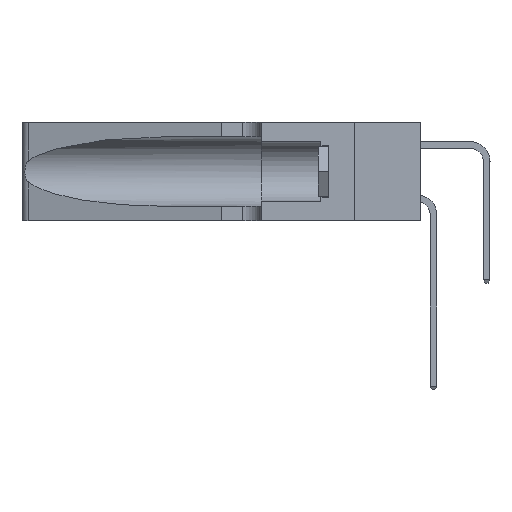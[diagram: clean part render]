
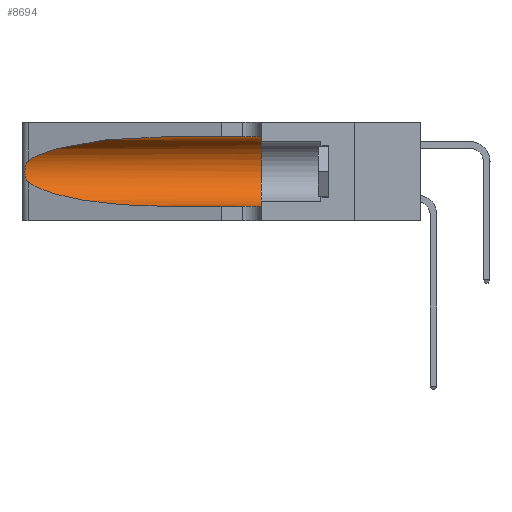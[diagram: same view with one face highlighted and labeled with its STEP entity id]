
A CAD part, left-side view. The second image highlights one B-rep face of the part: STEP entity #8694.
In plain terms, the highlighted cylindrical face has radius 3.308 mm (diameter 6.617 mm), a partial arc.
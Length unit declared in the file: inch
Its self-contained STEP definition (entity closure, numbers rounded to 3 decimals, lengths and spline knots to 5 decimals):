
#302 = EDGE_CURVE ( 'NONE', #23426, #15752, #14535, .T. ) ;
#501 = CARTESIAN_POINT ( 'NONE',  ( 0.18966, 0.96281, 0.31525 ) ) ;
#1126 = CARTESIAN_POINT ( 'NONE',  ( 0.25555, 1.22994, 0.2215 ) ) ;
#1220 = CARTESIAN_POINT ( 'NONE',  ( 0.25854, 1.2359, 0.20912 ) ) ;
#1507 = VECTOR ( 'NONE', #12776, 39.37008 ) ;
#2389 =( BOUNDED_CURVE ( )  B_SPLINE_CURVE ( 3, ( #27854, #23503, #28243, #2604 ),
 .UNSPECIFIED., .F., .T. ) 
 B_SPLINE_CURVE_WITH_KNOTS ( ( 4, 4 ),
 ( 3.44316, 4.71239 ),
 .UNSPECIFIED. ) 
 CURVE ( )  GEOMETRIC_REPRESENTATION_ITEM ( )  RATIONAL_B_SPLINE_CURVE ( ( 1., 0.87, 0.87, 1. ) ) 
 REPRESENTATION_ITEM ( '' )  );
#2604 = CARTESIAN_POINT ( 'NONE',  ( 0.1305, 0.72297, 0.05475 ) ) ;
#2962 = CARTESIAN_POINT ( 'NONE',  ( 0.1305, 0.72297, 0.31525 ) ) ;
#2973 = CYLINDRICAL_SURFACE ( 'NONE', #15668, 0.13025 ) ;
#3079 = CARTESIAN_POINT ( 'NONE',  ( 0.1305, 1.61858, 0.05475 ) ) ;
#3921 = EDGE_LOOP ( 'NONE', ( #8432, #19907, #19055, #15913, #11476, #18027 ) ) ;
#5424 = CARTESIAN_POINT ( 'NONE',  ( 0.25487, 1.22718, 0.22369 ) ) ;
#6348 = EDGE_CURVE ( 'NONE', #6691, #15752, #23844, .T. ) ;
#6691 = VERTEX_POINT ( 'NONE', #27721 ) ;
#7395 = CARTESIAN_POINT ( 'NONE',  ( 0.25487, 1.22718, 0.22369 ) ) ;
#7582 = CARTESIAN_POINT ( 'NONE',  ( 0.25487, 1.22718, 0.22369 ) ) ;
#8052 = DIRECTION ( 'NONE',  ( 0., -1., 0. ) ) ;
#8074 = CARTESIAN_POINT ( 'NONE',  ( 0.26018, 1.23835, 0.19895 ) ) ;
#8173 =( BOUNDED_CURVE ( )  B_SPLINE_CURVE ( 3, ( #2962, #501, #25653, #5424 ),
 .UNSPECIFIED., .F., .F. ) 
 B_SPLINE_CURVE_WITH_KNOTS ( ( 4, 4 ),
 ( 1.5708, 2.84003 ),
 .UNSPECIFIED. ) 
 CURVE ( )  GEOMETRIC_REPRESENTATION_ITEM ( )  RATIONAL_B_SPLINE_CURVE ( ( 1., 0.87, 0.87, 1. ) ) 
 REPRESENTATION_ITEM ( '' )  );
#8175 = CARTESIAN_POINT ( 'NONE',  ( 0.25555, 1.22993, 0.14849 ) ) ;
#8432 = ORIENTED_EDGE ( 'NONE', *, *, #15903, .T. ) ;
#8694 = ADVANCED_FACE ( 'NONE', ( #22070 ), #2973, .F. ) ;
#9464 = B_SPLINE_CURVE_WITH_KNOTS ( 'NONE', 3,
 ( #7582, #1126, #23892, #14987, #1220, #8074, #10182, #19201, #10084, #26168, #26359, #19395, #8175, #24179 ),
 .UNSPECIFIED., .F., .F.,
 ( 4, 2, 2, 2, 2, 2, 4 ),
 ( 0., 0.00027, 0.00053, 0.00107, 0.0016, 0.00187, 0.00214 ),
 .UNSPECIFIED. ) ;
#9949 = VERTEX_POINT ( 'NONE', #7395 ) ;
#10025 = CARTESIAN_POINT ( 'NONE',  ( 0.25487, 1.22718, 0.14631 ) ) ;
#10084 = CARTESIAN_POINT ( 'NONE',  ( 0.26017, 1.23833, 0.17102 ) ) ;
#10182 = CARTESIAN_POINT ( 'NONE',  ( 0.26075, 1.23896, 0.19203 ) ) ;
#10479 = CARTESIAN_POINT ( 'NONE',  ( 0.1305, 0.35, 0.185 ) ) ;
#10661 = DIRECTION ( 'NONE',  ( 0., 0., -1. ) ) ;
#11139 = VERTEX_POINT ( 'NONE', #17946 ) ;
#11476 = ORIENTED_EDGE ( 'NONE', *, *, #302, .F. ) ;
#11951 = EDGE_CURVE ( 'NONE', #19538, #6691, #2389, .T. ) ;
#12049 = EDGE_CURVE ( 'NONE', #9949, #19538, #9464, .T. ) ;
#12178 = DIRECTION ( 'NONE',  ( 0., -1., 0. ) ) ;
#12776 = DIRECTION ( 'NONE',  ( 0., -1., 0. ) ) ;
#14535 = CIRCLE ( 'NONE', #20336, 0.13025 ) ;
#14987 = CARTESIAN_POINT ( 'NONE',  ( 0.25787, 1.23484, 0.2124 ) ) ;
#15668 = AXIS2_PLACEMENT_3D ( 'NONE', #18980, #8052, #10661 ) ;
#15752 = VERTEX_POINT ( 'NONE', #18091 ) ;
#15903 = EDGE_CURVE ( 'NONE', #11139, #9949, #8173, .T. ) ;
#15913 = ORIENTED_EDGE ( 'NONE', *, *, #6348, .T. ) ;
#17285 = CARTESIAN_POINT ( 'NONE',  ( 0.1305, 1.61858, 0.31525 ) ) ;
#17946 = CARTESIAN_POINT ( 'NONE',  ( 0.1305, 0.72297, 0.31525 ) ) ;
#18027 = ORIENTED_EDGE ( 'NONE', *, *, #25657, .F. ) ;
#18091 = CARTESIAN_POINT ( 'NONE',  ( 0.1305, 0.35, 0.05475 ) ) ;
#18748 = LINE ( 'NONE', #17285, #1507 ) ;
#18980 = CARTESIAN_POINT ( 'NONE',  ( 0.1305, 1.61858, 0.185 ) ) ;
#19055 = ORIENTED_EDGE ( 'NONE', *, *, #11951, .T. ) ;
#19201 = CARTESIAN_POINT ( 'NONE',  ( 0.26075, 1.23896, 0.178 ) ) ;
#19395 = CARTESIAN_POINT ( 'NONE',  ( 0.25639, 1.23186, 0.15144 ) ) ;
#19495 = DIRECTION ( 'NONE',  ( 0., 1., 0. ) ) ;
#19538 = VERTEX_POINT ( 'NONE', #10025 ) ;
#19546 = VECTOR ( 'NONE', #12178, 39.37008 ) ;
#19889 = DIRECTION ( 'NONE',  ( 0., 0., 1. ) ) ;
#19907 = ORIENTED_EDGE ( 'NONE', *, *, #12049, .T. ) ;
#20336 = AXIS2_PLACEMENT_3D ( 'NONE', #10479, #19495, #19889 ) ;
#22070 = FACE_OUTER_BOUND ( 'NONE', #3921, .T. ) ;
#23426 = VERTEX_POINT ( 'NONE', #28849 ) ;
#23503 = CARTESIAN_POINT ( 'NONE',  ( 0.2373, 1.15595, 0.08982 ) ) ;
#23844 = LINE ( 'NONE', #3079, #19546 ) ;
#23892 = CARTESIAN_POINT ( 'NONE',  ( 0.25639, 1.23184, 0.21858 ) ) ;
#24179 = CARTESIAN_POINT ( 'NONE',  ( 0.25487, 1.22718, 0.14631 ) ) ;
#25653 = CARTESIAN_POINT ( 'NONE',  ( 0.2373, 1.15595, 0.28018 ) ) ;
#25657 = EDGE_CURVE ( 'NONE', #11139, #23426, #18748, .T. ) ;
#26168 = CARTESIAN_POINT ( 'NONE',  ( 0.25856, 1.23593, 0.16098 ) ) ;
#26359 = CARTESIAN_POINT ( 'NONE',  ( 0.25789, 1.23486, 0.15765 ) ) ;
#27721 = CARTESIAN_POINT ( 'NONE',  ( 0.1305, 0.72297, 0.05475 ) ) ;
#27854 = CARTESIAN_POINT ( 'NONE',  ( 0.25487, 1.22718, 0.14631 ) ) ;
#28243 = CARTESIAN_POINT ( 'NONE',  ( 0.18966, 0.96281, 0.05475 ) ) ;
#28849 = CARTESIAN_POINT ( 'NONE',  ( 0.1305, 0.35, 0.31525 ) ) ;
